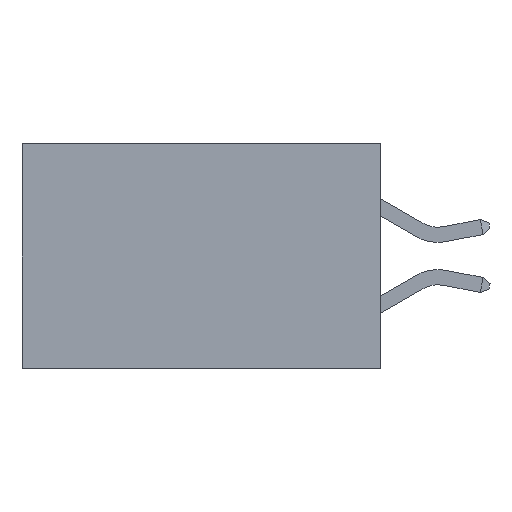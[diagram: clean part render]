
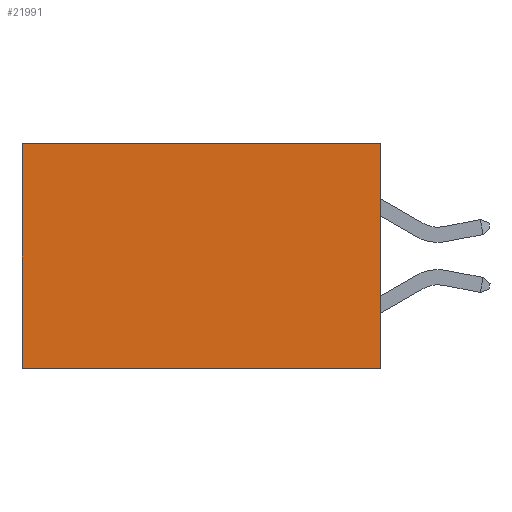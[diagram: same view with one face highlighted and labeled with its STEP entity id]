
A CAD part, left-side view. The second image highlights one B-rep face of the part: STEP entity #21991.
In plain terms, the highlighted planar face has unit normal (-1, 0, 0).
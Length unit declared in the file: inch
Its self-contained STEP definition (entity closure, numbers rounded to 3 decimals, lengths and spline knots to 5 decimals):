
#796 = FACE_OUTER_BOUND ( 'NONE', #17784, .T. ) ;
#1237 = CARTESIAN_POINT ( 'NONE',  ( 0.277, 0., -0.37 ) ) ;
#1350 = EDGE_CURVE ( 'NONE', #19616, #8946, #18924, .T. ) ;
#1578 = CARTESIAN_POINT ( 'NONE',  ( 0.277, 0.59, -0.37 ) ) ;
#2008 = CARTESIAN_POINT ( 'NONE',  ( 0.277, 0.59, 0. ) ) ;
#2428 = DIRECTION ( 'NONE',  ( 0., 1., 0. ) ) ;
#2484 = LINE ( 'NONE', #12147, #11385 ) ;
#3309 = DIRECTION ( 'NONE',  ( 0., 0., -1. ) ) ;
#3561 = DIRECTION ( 'NONE',  ( 1., 0., 0. ) ) ;
#3982 = ORIENTED_EDGE ( 'NONE', *, *, #7545, .T. ) ;
#4550 = EDGE_CURVE ( 'NONE', #20163, #8946, #2484, .T. ) ;
#4644 = LINE ( 'NONE', #9495, #18168 ) ;
#4914 = VERTEX_POINT ( 'NONE', #7882 ) ;
#5177 = DIRECTION ( 'NONE',  ( 0., 0., -1. ) ) ;
#6044 = EDGE_CURVE ( 'NONE', #4914, #20163, #18462, .T. ) ;
#6512 = ORIENTED_EDGE ( 'NONE', *, *, #1350, .T. ) ;
#7545 = EDGE_CURVE ( 'NONE', #4914, #19616, #4644, .T. ) ;
#7882 = CARTESIAN_POINT ( 'NONE',  ( 0.277, 0., 0. ) ) ;
#8189 = ORIENTED_EDGE ( 'NONE', *, *, #6044, .F. ) ;
#8946 = VERTEX_POINT ( 'NONE', #11154 ) ;
#9495 = CARTESIAN_POINT ( 'NONE',  ( 0.277, 0., 0. ) ) ;
#11154 = CARTESIAN_POINT ( 'NONE',  ( 0.277, 0.59, -0.37 ) ) ;
#11272 = AXIS2_PLACEMENT_3D ( 'NONE', #14163, #3561, #15956 ) ;
#11385 = VECTOR ( 'NONE', #16076, 39.37008 ) ;
#11762 = ORIENTED_EDGE ( 'NONE', *, *, #4550, .F. ) ;
#12147 = CARTESIAN_POINT ( 'NONE',  ( 0.277, 0., -0.37 ) ) ;
#14163 = CARTESIAN_POINT ( 'NONE',  ( 0.277, 0., -0.37 ) ) ;
#14237 = VECTOR ( 'NONE', #5177, 39.37008 ) ;
#15937 = CARTESIAN_POINT ( 'NONE',  ( 0.277, 0., -0.37 ) ) ;
#15956 = DIRECTION ( 'NONE',  ( 0., 0., -1. ) ) ;
#16076 = DIRECTION ( 'NONE',  ( 0., 1., 0. ) ) ;
#17361 = VECTOR ( 'NONE', #3309, 39.37008 ) ;
#17498 = PLANE ( 'NONE',  #11272 ) ;
#17784 = EDGE_LOOP ( 'NONE', ( #6512, #11762, #8189, #3982 ) ) ;
#18168 = VECTOR ( 'NONE', #2428, 39.37008 ) ;
#18462 = LINE ( 'NONE', #1237, #17361 ) ;
#18924 = LINE ( 'NONE', #1578, #14237 ) ;
#19616 = VERTEX_POINT ( 'NONE', #2008 ) ;
#20163 = VERTEX_POINT ( 'NONE', #15937 ) ;
#21991 = ADVANCED_FACE ( 'NONE', ( #796 ), #17498, .F. ) ;
